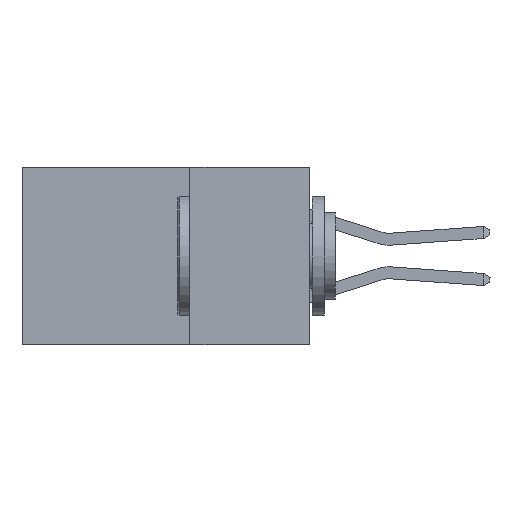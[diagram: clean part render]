
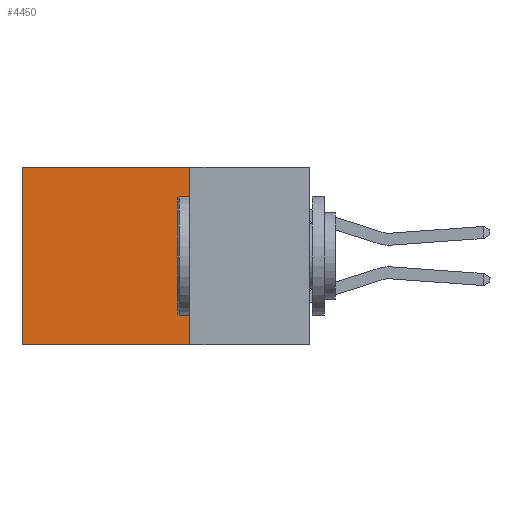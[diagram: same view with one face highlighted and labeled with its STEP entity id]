
A CAD part, left-side view. The second image highlights one B-rep face of the part: STEP entity #4450.
In plain terms, the highlighted planar face has unit normal (-1, 0, 0).
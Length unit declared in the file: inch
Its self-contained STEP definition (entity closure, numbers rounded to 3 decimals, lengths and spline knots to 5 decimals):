
#287 = PLANE ( 'NONE',  #5476 ) ;
#670 = VECTOR ( 'NONE', #2988, 39.37008 ) ;
#1086 = ORIENTED_EDGE ( 'NONE', *, *, #9507, .F. ) ;
#1727 = CARTESIAN_POINT ( 'NONE',  ( 0.2615, 0.25, -0.37 ) ) ;
#1856 = DIRECTION ( 'NONE',  ( 0., 0., -1. ) ) ;
#2988 = DIRECTION ( 'NONE',  ( 0., 0., -1. ) ) ;
#4076 = DIRECTION ( 'NONE',  ( 0., 1., 0. ) ) ;
#4271 = DIRECTION ( 'NONE',  ( 0., 1., 0. ) ) ;
#4321 = LINE ( 'NONE', #15096, #670 ) ;
#4450 = ADVANCED_FACE ( 'NONE', ( #17963 ), #287, .F. ) ;
#4504 = EDGE_CURVE ( 'NONE', #6593, #12499, #5039, .T. ) ;
#4791 = CARTESIAN_POINT ( 'NONE',  ( 0.2615, 0.6, -0.37 ) ) ;
#4793 = ORIENTED_EDGE ( 'NONE', *, *, #4504, .F. ) ;
#5039 = LINE ( 'NONE', #5089, #9135 ) ;
#5089 = CARTESIAN_POINT ( 'NONE',  ( 0.2615, 0.25, -0.37 ) ) ;
#5476 = AXIS2_PLACEMENT_3D ( 'NONE', #18413, #11020, #1856 ) ;
#6140 = LINE ( 'NONE', #16135, #17626 ) ;
#6593 = VERTEX_POINT ( 'NONE', #14063 ) ;
#6890 = EDGE_CURVE ( 'NONE', #6593, #10257, #6140, .T. ) ;
#7777 = VERTEX_POINT ( 'NONE', #4791 ) ;
#9007 = EDGE_LOOP ( 'NONE', ( #11360, #1086, #4793, #15621 ) ) ;
#9135 = VECTOR ( 'NONE', #15630, 39.37008 ) ;
#9507 = EDGE_CURVE ( 'NONE', #12499, #7777, #12406, .T. ) ;
#10257 = VERTEX_POINT ( 'NONE', #11936 ) ;
#10338 = CARTESIAN_POINT ( 'NONE',  ( 0.2615, 0.25, -0.37 ) ) ;
#11020 = DIRECTION ( 'NONE',  ( 1., 0., 0. ) ) ;
#11360 = ORIENTED_EDGE ( 'NONE', *, *, #11814, .T. ) ;
#11814 = EDGE_CURVE ( 'NONE', #10257, #7777, #4321, .T. ) ;
#11936 = CARTESIAN_POINT ( 'NONE',  ( 0.2615, 0.6, 0. ) ) ;
#12406 = LINE ( 'NONE', #10338, #15910 ) ;
#12499 = VERTEX_POINT ( 'NONE', #1727 ) ;
#14063 = CARTESIAN_POINT ( 'NONE',  ( 0.2615, 0.25, 0. ) ) ;
#15096 = CARTESIAN_POINT ( 'NONE',  ( 0.2615, 0.6, -0.37 ) ) ;
#15621 = ORIENTED_EDGE ( 'NONE', *, *, #6890, .T. ) ;
#15630 = DIRECTION ( 'NONE',  ( 0., 0., -1. ) ) ;
#15910 = VECTOR ( 'NONE', #4271, 39.37008 ) ;
#16135 = CARTESIAN_POINT ( 'NONE',  ( 0.2615, 0.25, 0. ) ) ;
#17626 = VECTOR ( 'NONE', #4076, 39.37008 ) ;
#17963 = FACE_OUTER_BOUND ( 'NONE', #9007, .T. ) ;
#18413 = CARTESIAN_POINT ( 'NONE',  ( 0.2615, 0.25, -0.37 ) ) ;
